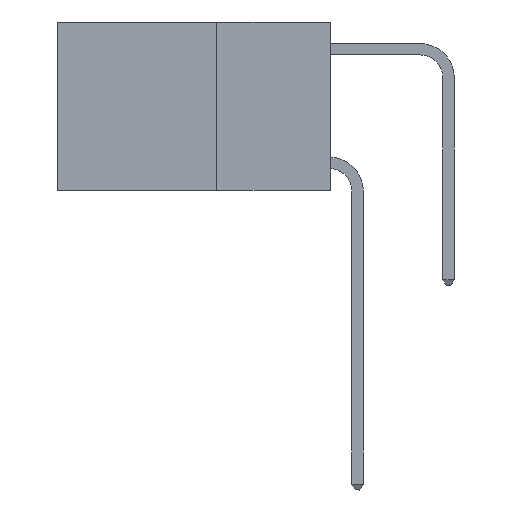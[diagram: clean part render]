
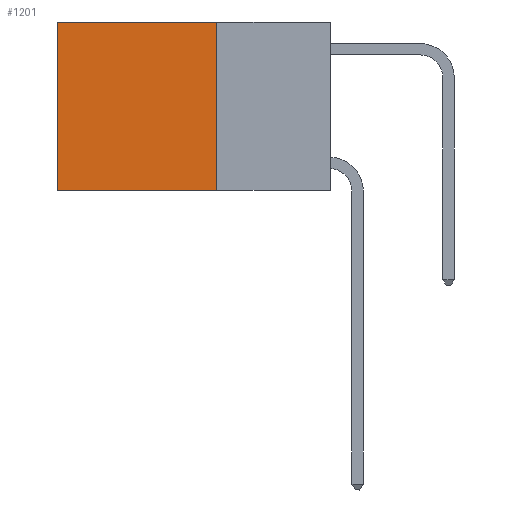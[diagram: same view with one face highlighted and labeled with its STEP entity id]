
A CAD part, left-side view. The second image highlights one B-rep face of the part: STEP entity #1201.
In plain terms, the highlighted planar face has unit normal (-1, 0, 0).
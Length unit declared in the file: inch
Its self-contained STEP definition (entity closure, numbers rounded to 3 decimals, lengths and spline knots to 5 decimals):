
#461 = CARTESIAN_POINT ( 'NONE',  ( 0.2625, 0.25, -0.37 ) ) ;
#750 = LINE ( 'NONE', #10540, #18495 ) ;
#1201 = ADVANCED_FACE ( 'NONE', ( #23581 ), #14438, .F. ) ;
#2658 = VECTOR ( 'NONE', #5784, 39.37008 ) ;
#5203 = DIRECTION ( 'NONE',  ( 0., 0., -1. ) ) ;
#5784 = DIRECTION ( 'NONE',  ( 0., 1., 0. ) ) ;
#6760 = DIRECTION ( 'NONE',  ( 1., 0., 0. ) ) ;
#7193 = EDGE_CURVE ( 'NONE', #12974, #16637, #23551, .T. ) ;
#8139 = CARTESIAN_POINT ( 'NONE',  ( 0.2625, 0.6, 0. ) ) ;
#9266 = CARTESIAN_POINT ( 'NONE',  ( 0.2625, 0.6, 0. ) ) ;
#9499 = EDGE_CURVE ( 'NONE', #16637, #15830, #11865, .T. ) ;
#10540 = CARTESIAN_POINT ( 'NONE',  ( 0.2625, 0.25, -0.37 ) ) ;
#11865 = LINE ( 'NONE', #8139, #15580 ) ;
#11886 = DIRECTION ( 'NONE',  ( 0., 0., -1. ) ) ;
#12394 = DIRECTION ( 'NONE',  ( 0., 1., 0. ) ) ;
#12934 = EDGE_LOOP ( 'NONE', ( #17297, #18726, #15519, #15265 ) ) ;
#12974 = VERTEX_POINT ( 'NONE', #18264 ) ;
#14438 = PLANE ( 'NONE',  #19216 ) ;
#14512 = CARTESIAN_POINT ( 'NONE',  ( 0.2625, 0.25, 0. ) ) ;
#15265 = ORIENTED_EDGE ( 'NONE', *, *, #7193, .T. ) ;
#15330 = LINE ( 'NONE', #23477, #21385 ) ;
#15519 = ORIENTED_EDGE ( 'NONE', *, *, #22577, .F. ) ;
#15580 = VECTOR ( 'NONE', #11886, 39.37008 ) ;
#15830 = VERTEX_POINT ( 'NONE', #22386 ) ;
#16637 = VERTEX_POINT ( 'NONE', #9266 ) ;
#17297 = ORIENTED_EDGE ( 'NONE', *, *, #9499, .T. ) ;
#18264 = CARTESIAN_POINT ( 'NONE',  ( 0.2625, 0.25, 0. ) ) ;
#18495 = VECTOR ( 'NONE', #12394, 39.37008 ) ;
#18726 = ORIENTED_EDGE ( 'NONE', *, *, #23661, .F. ) ;
#19216 = AXIS2_PLACEMENT_3D ( 'NONE', #14512, #6760, #5203 ) ;
#21385 = VECTOR ( 'NONE', #24044, 39.37008 ) ;
#22214 = CARTESIAN_POINT ( 'NONE',  ( 0.2625, 0.25, 0. ) ) ;
#22386 = CARTESIAN_POINT ( 'NONE',  ( 0.2625, 0.6, -0.37 ) ) ;
#22577 = EDGE_CURVE ( 'NONE', #12974, #23392, #15330, .T. ) ;
#23392 = VERTEX_POINT ( 'NONE', #461 ) ;
#23477 = CARTESIAN_POINT ( 'NONE',  ( 0.2625, 0.25, 0. ) ) ;
#23551 = LINE ( 'NONE', #22214, #2658 ) ;
#23581 = FACE_OUTER_BOUND ( 'NONE', #12934, .T. ) ;
#23661 = EDGE_CURVE ( 'NONE', #23392, #15830, #750, .T. ) ;
#24044 = DIRECTION ( 'NONE',  ( 0., 0., -1. ) ) ;
